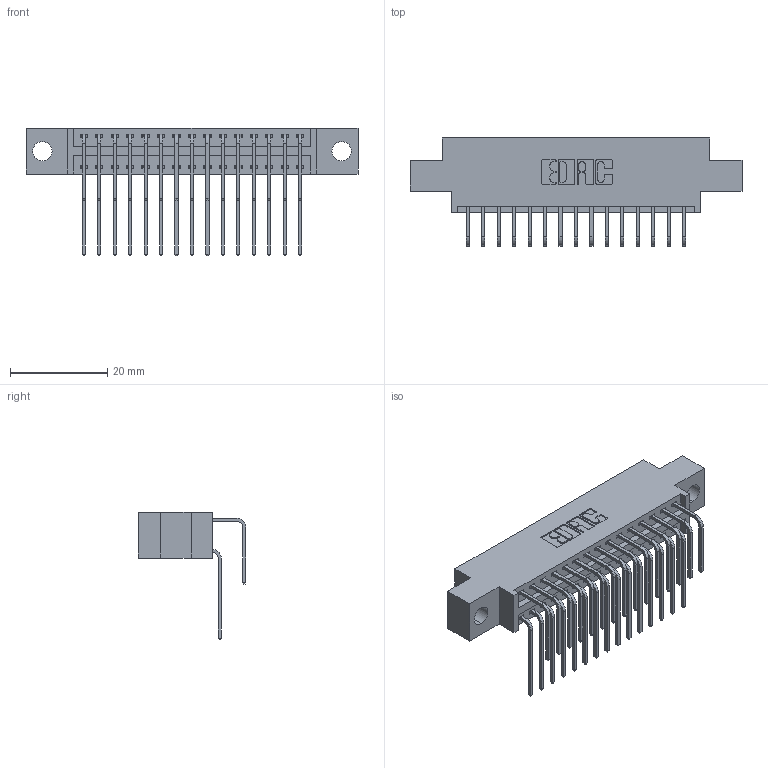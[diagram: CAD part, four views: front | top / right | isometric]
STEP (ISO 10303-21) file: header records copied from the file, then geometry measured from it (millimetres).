
FILE_DESCRIPTION (( 'STEP AP203' ), '1' );
FILE_NAME ('346-030-558-804.STEP', '2022-05-19T17:01:34', ( '' ), ( '' ), 'SwSTEP 2.0', 'SolidWorks 2020', '' );
FILE_SCHEMA (( 'CONFIG_CONTROL_DESIGN' ));
Length unit declared in the file: inch
Products named in the file (4): 346-030-558-804; 345-292-001_558 Tail - 2; 345-292-001_558 559 Tail - 1; 346 Part_0.170 Offset - 0.156 Dia-TH
Assembly tree (31 placements, depth 2):
  346-030-558-804
    346 Part_0.170 Offset - 0.156 Dia-TH
    345-292-001_558 559 Tail - 1  x15
    345-292-001_558 Tail - 2  x15
Bounding box: 68.2 x 22.16 x 26.16 mm (x, y, z)
Volume: 6353 mm3; surface area: 9166.1 mm2
Topology: 31 solids, 31 shells, 1760 faces, 5207 edges, 3430 vertices
Faces by surface type: plane 1204, cylinder 556
Entity records: 15759 total; most frequent: CARTESIAN_POINT 2693, ORIENTED_EDGE 2574, DIRECTION 2395, EDGE_CURVE 1287, LINE 1055, VECTOR 1055, VERTEX_POINT 854, AXIS2_PLACEMENT_3D 670
